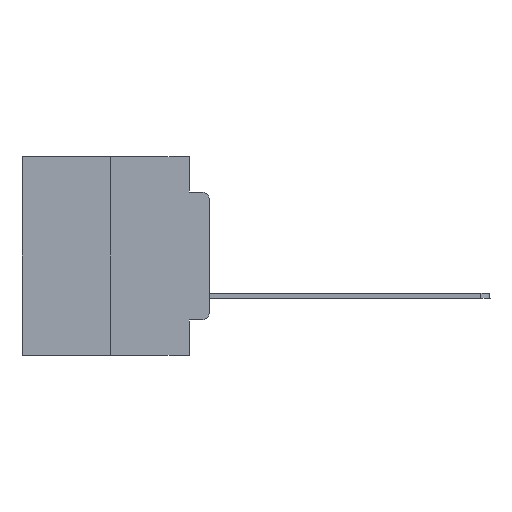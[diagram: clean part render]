
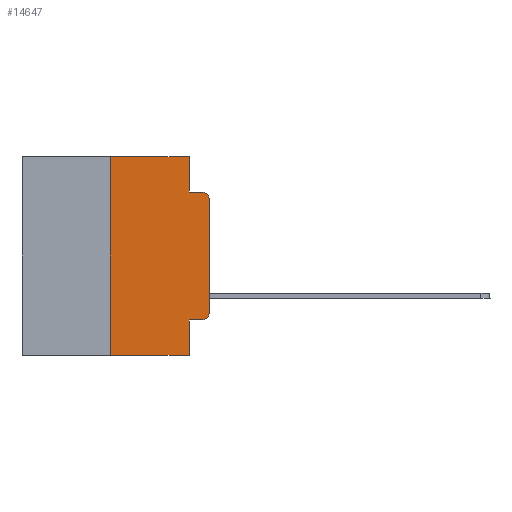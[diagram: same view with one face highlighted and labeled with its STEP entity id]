
A CAD part, left-side view. The second image highlights one B-rep face of the part: STEP entity #14647.
In plain terms, the highlighted planar face has unit normal (-1, 0, 0).
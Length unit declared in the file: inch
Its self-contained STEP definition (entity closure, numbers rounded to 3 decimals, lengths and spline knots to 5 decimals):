
#400 = EDGE_LOOP ( 'NONE', ( #23851, #2469, #22181, #23230, #13097, #20881, #8729, #25815, #6090, #1468 ) ) ;
#1355 = VECTOR ( 'NONE', #5261, 39.37008 ) ;
#1468 = ORIENTED_EDGE ( 'NONE', *, *, #16766, .T. ) ;
#1884 = CARTESIAN_POINT ( 'NONE',  ( 0., 0.473, -0.5 ) ) ;
#2030 = LINE ( 'NONE', #1884, #23041 ) ;
#2103 = VERTEX_POINT ( 'NONE', #26498 ) ;
#2421 = EDGE_CURVE ( 'NONE', #2103, #19887, #3195, .T. ) ;
#2469 = ORIENTED_EDGE ( 'NONE', *, *, #24408, .T. ) ;
#3195 = LINE ( 'NONE', #24178, #5191 ) ;
#3596 = DIRECTION ( 'NONE',  ( 1., 0., 0. ) ) ;
#4097 = EDGE_CURVE ( 'NONE', #23070, #19531, #12313, .T. ) ;
#4247 = VERTEX_POINT ( 'NONE', #26224 ) ;
#4316 = FACE_OUTER_BOUND ( 'NONE', #400, .T. ) ;
#4373 = CIRCLE ( 'NONE', #4783, 0.02 ) ;
#4375 = CARTESIAN_POINT ( 'NONE',  ( 0., 0.051, 0. ) ) ;
#4498 = DIRECTION ( 'NONE',  ( 0., 0., -1. ) ) ;
#4783 = AXIS2_PLACEMENT_3D ( 'NONE', #21715, #21458, #4498 ) ;
#5191 = VECTOR ( 'NONE', #11272, 39.37008 ) ;
#5261 = DIRECTION ( 'NONE',  ( 0., 0., 1. ) ) ;
#6090 = ORIENTED_EDGE ( 'NONE', *, *, #2421, .T. ) ;
#6826 = AXIS2_PLACEMENT_3D ( 'NONE', #12200, #14455, #21071 ) ;
#7052 = CARTESIAN_POINT ( 'NONE',  ( 0., 0.25, -0.5 ) ) ;
#7091 = CIRCLE ( 'NONE', #6826, 0.02 ) ;
#7525 = VERTEX_POINT ( 'NONE', #7052 ) ;
#7869 = CARTESIAN_POINT ( 'NONE',  ( 0., 0.051, 0. ) ) ;
#7960 = EDGE_CURVE ( 'NONE', #8351, #4247, #12427, .T. ) ;
#8201 = VERTEX_POINT ( 'NONE', #26560 ) ;
#8351 = VERTEX_POINT ( 'NONE', #16102 ) ;
#8729 = ORIENTED_EDGE ( 'NONE', *, *, #17614, .T. ) ;
#8941 = VECTOR ( 'NONE', #16760, 39.37008 ) ;
#9572 = CARTESIAN_POINT ( 'NONE',  ( 0., 0., -0.3915 ) ) ;
#10295 = EDGE_CURVE ( 'NONE', #4247, #18973, #16534, .T. ) ;
#11039 = EDGE_CURVE ( 'NONE', #8201, #8351, #20849, .T. ) ;
#11272 = DIRECTION ( 'NONE',  ( 0., -1., 0. ) ) ;
#11372 = CARTESIAN_POINT ( 'NONE',  ( 0., 0.473, 0. ) ) ;
#11427 = CARTESIAN_POINT ( 'NONE',  ( 0., 0.25, 0. ) ) ;
#11632 = VECTOR ( 'NONE', #15973, 39.37008 ) ;
#12200 = CARTESIAN_POINT ( 'NONE',  ( 0., 0.02, -0.1085 ) ) ;
#12313 = LINE ( 'NONE', #18474, #11632 ) ;
#12427 = LINE ( 'NONE', #4375, #15769 ) ;
#12497 = CARTESIAN_POINT ( 'NONE',  ( 0., 0.051, -0.0885 ) ) ;
#12663 = DIRECTION ( 'NONE',  ( 0., 0., -1. ) ) ;
#13097 = ORIENTED_EDGE ( 'NONE', *, *, #11039, .F. ) ;
#13643 = EDGE_CURVE ( 'NONE', #7525, #8201, #25636, .T. ) ;
#14455 = DIRECTION ( 'NONE',  ( -1., 0., 0. ) ) ;
#14647 = ADVANCED_FACE ( 'NONE', ( #4316 ), #24820, .F. ) ;
#14762 = DIRECTION ( 'NONE',  ( 0., -1., 0. ) ) ;
#14818 = CARTESIAN_POINT ( 'NONE',  ( 0., 0.02, -0.0885 ) ) ;
#15571 = CARTESIAN_POINT ( 'NONE',  ( 0., 0.02, -0.4115 ) ) ;
#15769 = VECTOR ( 'NONE', #12663, 39.37008 ) ;
#15973 = DIRECTION ( 'NONE',  ( 0., 0., 1. ) ) ;
#16027 = AXIS2_PLACEMENT_3D ( 'NONE', #26922, #3596, #16548 ) ;
#16102 = CARTESIAN_POINT ( 'NONE',  ( 0., 0.051, 0. ) ) ;
#16534 = LINE ( 'NONE', #12497, #19210 ) ;
#16548 = DIRECTION ( 'NONE',  ( 0., 0., -1. ) ) ;
#16760 = DIRECTION ( 'NONE',  ( 0., 0., -1. ) ) ;
#16766 = EDGE_CURVE ( 'NONE', #19887, #23070, #4373, .T. ) ;
#17614 = EDGE_CURVE ( 'NONE', #7525, #26546, #2030, .T. ) ;
#17863 = EDGE_CURVE ( 'NONE', #2103, #26546, #20009, .T. ) ;
#18474 = CARTESIAN_POINT ( 'NONE',  ( 0., 0., 0. ) ) ;
#18973 = VERTEX_POINT ( 'NONE', #14818 ) ;
#19210 = VECTOR ( 'NONE', #25421, 39.37008 ) ;
#19531 = VERTEX_POINT ( 'NONE', #27260 ) ;
#19678 = DIRECTION ( 'NONE',  ( 0., -1., 0. ) ) ;
#19887 = VERTEX_POINT ( 'NONE', #15571 ) ;
#20009 = LINE ( 'NONE', #7869, #8941 ) ;
#20849 = LINE ( 'NONE', #11372, #22858 ) ;
#20881 = ORIENTED_EDGE ( 'NONE', *, *, #13643, .F. ) ;
#21071 = DIRECTION ( 'NONE',  ( 0., 0., -1. ) ) ;
#21458 = DIRECTION ( 'NONE',  ( -1., 0., 0. ) ) ;
#21715 = CARTESIAN_POINT ( 'NONE',  ( 0., 0.02, -0.3915 ) ) ;
#22181 = ORIENTED_EDGE ( 'NONE', *, *, #10295, .F. ) ;
#22858 = VECTOR ( 'NONE', #19678, 39.37008 ) ;
#23041 = VECTOR ( 'NONE', #14762, 39.37008 ) ;
#23070 = VERTEX_POINT ( 'NONE', #9572 ) ;
#23230 = ORIENTED_EDGE ( 'NONE', *, *, #7960, .F. ) ;
#23573 = CARTESIAN_POINT ( 'NONE',  ( 0., 0.051, -0.5 ) ) ;
#23851 = ORIENTED_EDGE ( 'NONE', *, *, #4097, .T. ) ;
#24178 = CARTESIAN_POINT ( 'NONE',  ( 0., 0.051, -0.4115 ) ) ;
#24408 = EDGE_CURVE ( 'NONE', #19531, #18973, #7091, .T. ) ;
#24820 = PLANE ( 'NONE',  #16027 ) ;
#25421 = DIRECTION ( 'NONE',  ( 0., -1., 0. ) ) ;
#25636 = LINE ( 'NONE', #11427, #1355 ) ;
#25815 = ORIENTED_EDGE ( 'NONE', *, *, #17863, .F. ) ;
#26224 = CARTESIAN_POINT ( 'NONE',  ( 0., 0.051, -0.0885 ) ) ;
#26498 = CARTESIAN_POINT ( 'NONE',  ( 0., 0.051, -0.4115 ) ) ;
#26546 = VERTEX_POINT ( 'NONE', #23573 ) ;
#26560 = CARTESIAN_POINT ( 'NONE',  ( 0., 0.25, 0. ) ) ;
#26922 = CARTESIAN_POINT ( 'NONE',  ( 0., 0.473, 0. ) ) ;
#27260 = CARTESIAN_POINT ( 'NONE',  ( 0., 0., -0.1085 ) ) ;
